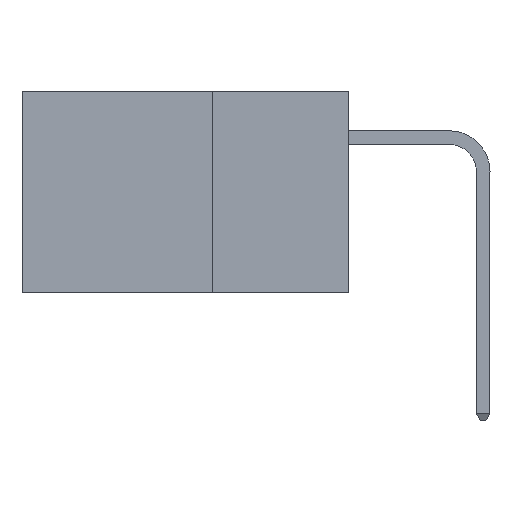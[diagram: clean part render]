
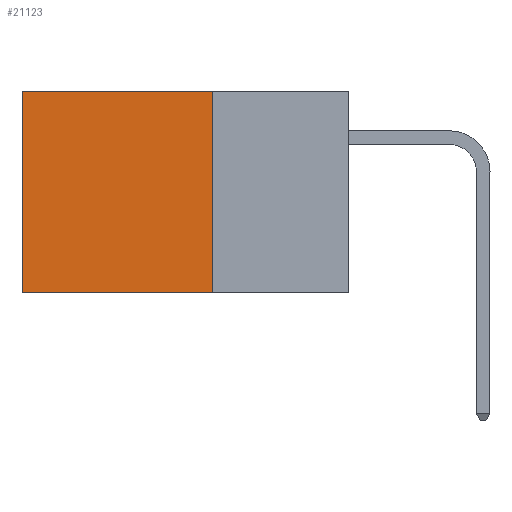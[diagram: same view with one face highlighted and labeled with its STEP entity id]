
A CAD part, left-side view. The second image highlights one B-rep face of the part: STEP entity #21123.
In plain terms, the highlighted planar face has unit normal (-1, 0, 0).
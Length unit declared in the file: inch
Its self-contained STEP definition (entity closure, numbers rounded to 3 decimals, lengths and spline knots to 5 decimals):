
#1730 = CARTESIAN_POINT ( 'NONE',  ( 0.2875, 0.25, 0. ) ) ;
#1898 = DIRECTION ( 'NONE',  ( 0., 0., -1. ) ) ;
#2970 = VECTOR ( 'NONE', #4405, 39.37008 ) ;
#3021 = EDGE_CURVE ( 'NONE', #6184, #12428, #21001, .T. ) ;
#3057 = VERTEX_POINT ( 'NONE', #1730 ) ;
#3386 = DIRECTION ( 'NONE',  ( 0., 1., 0. ) ) ;
#3614 = CARTESIAN_POINT ( 'NONE',  ( 0.2875, 0.6, -0.37 ) ) ;
#3757 = LINE ( 'NONE', #6949, #21125 ) ;
#4405 = DIRECTION ( 'NONE',  ( 0., 1., 0. ) ) ;
#4514 = CARTESIAN_POINT ( 'NONE',  ( 0.2875, 0.6, 0. ) ) ;
#5370 = PLANE ( 'NONE',  #14609 ) ;
#5462 = EDGE_CURVE ( 'NONE', #3057, #12755, #20878, .T. ) ;
#6184 = VERTEX_POINT ( 'NONE', #15201 ) ;
#6949 = CARTESIAN_POINT ( 'NONE',  ( 0.2875, 0.25, 0. ) ) ;
#7064 = VECTOR ( 'NONE', #3386, 39.37008 ) ;
#8774 = DIRECTION ( 'NONE',  ( 1., 0., 0. ) ) ;
#9432 = CARTESIAN_POINT ( 'NONE',  ( 0.2875, 0.25, 0. ) ) ;
#9897 = ORIENTED_EDGE ( 'NONE', *, *, #10726, .F. ) ;
#10179 = FACE_OUTER_BOUND ( 'NONE', #15377, .T. ) ;
#10240 = LINE ( 'NONE', #4514, #18091 ) ;
#10726 = EDGE_CURVE ( 'NONE', #3057, #6184, #3757, .T. ) ;
#10748 = ORIENTED_EDGE ( 'NONE', *, *, #3021, .F. ) ;
#11309 = CARTESIAN_POINT ( 'NONE',  ( 0.2875, 0.6, 0. ) ) ;
#11830 = CARTESIAN_POINT ( 'NONE',  ( 0.2875, 0.25, -0.37 ) ) ;
#12428 = VERTEX_POINT ( 'NONE', #3614 ) ;
#12755 = VERTEX_POINT ( 'NONE', #11309 ) ;
#13257 = ORIENTED_EDGE ( 'NONE', *, *, #5462, .T. ) ;
#14609 = AXIS2_PLACEMENT_3D ( 'NONE', #15484, #8774, #20507 ) ;
#14638 = DIRECTION ( 'NONE',  ( 0., 0., -1. ) ) ;
#15201 = CARTESIAN_POINT ( 'NONE',  ( 0.2875, 0.25, -0.37 ) ) ;
#15377 = EDGE_LOOP ( 'NONE', ( #18061, #10748, #9897, #13257 ) ) ;
#15484 = CARTESIAN_POINT ( 'NONE',  ( 0.2875, 0.25, 0. ) ) ;
#18061 = ORIENTED_EDGE ( 'NONE', *, *, #18184, .T. ) ;
#18091 = VECTOR ( 'NONE', #14638, 39.37008 ) ;
#18184 = EDGE_CURVE ( 'NONE', #12755, #12428, #10240, .T. ) ;
#20507 = DIRECTION ( 'NONE',  ( 0., 0., -1. ) ) ;
#20878 = LINE ( 'NONE', #9432, #2970 ) ;
#21001 = LINE ( 'NONE', #11830, #7064 ) ;
#21123 = ADVANCED_FACE ( 'NONE', ( #10179 ), #5370, .F. ) ;
#21125 = VECTOR ( 'NONE', #1898, 39.37008 ) ;
